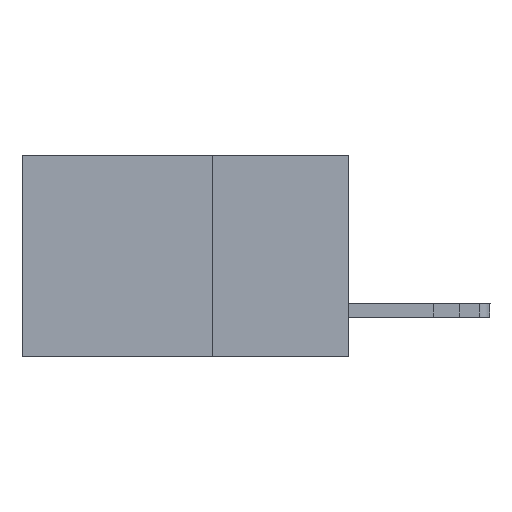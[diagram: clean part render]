
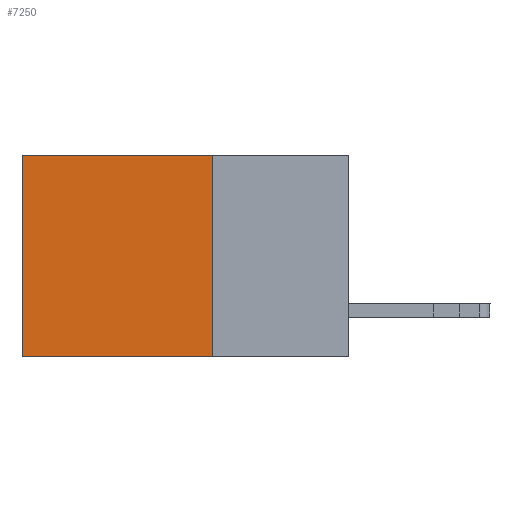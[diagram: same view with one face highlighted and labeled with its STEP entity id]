
A CAD part, left-side view. The second image highlights one B-rep face of the part: STEP entity #7250.
In plain terms, the highlighted planar face has unit normal (-1, 0, 0).
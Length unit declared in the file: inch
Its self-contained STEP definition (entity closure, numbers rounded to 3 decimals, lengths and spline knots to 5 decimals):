
#234 = DIRECTION ( 'NONE',  ( 0., 0., -1. ) ) ;
#355 = VERTEX_POINT ( 'NONE', #6419 ) ;
#730 = ORIENTED_EDGE ( 'NONE', *, *, #4278, .F. ) ;
#1530 = CARTESIAN_POINT ( 'NONE',  ( 0.2615, 0.25, -0.37 ) ) ;
#1921 = CARTESIAN_POINT ( 'NONE',  ( 0.2615, 0.25, 0. ) ) ;
#2441 = AXIS2_PLACEMENT_3D ( 'NONE', #8432, #5954, #5156 ) ;
#2687 = LINE ( 'NONE', #1921, #5431 ) ;
#2782 = PLANE ( 'NONE',  #2441 ) ;
#2874 = FACE_OUTER_BOUND ( 'NONE', #3683, .T. ) ;
#2915 = VECTOR ( 'NONE', #6944, 39.37008 ) ;
#3198 = VECTOR ( 'NONE', #234, 39.37008 ) ;
#3479 = CARTESIAN_POINT ( 'NONE',  ( 0.2615, 0.6, 0. ) ) ;
#3683 = EDGE_LOOP ( 'NONE', ( #8567, #730, #8002, #8547 ) ) ;
#3922 = CARTESIAN_POINT ( 'NONE',  ( 0.2615, 0.25, -0.37 ) ) ;
#3993 = EDGE_CURVE ( 'NONE', #6884, #7990, #2687, .T. ) ;
#4278 = EDGE_CURVE ( 'NONE', #5922, #355, #8503, .T. ) ;
#4698 = EDGE_CURVE ( 'NONE', #6884, #5922, #4733, .T. ) ;
#4733 = LINE ( 'NONE', #1530, #2915 ) ;
#4988 = LINE ( 'NONE', #8118, #3198 ) ;
#5156 = DIRECTION ( 'NONE',  ( 0., 0., -1. ) ) ;
#5431 = VECTOR ( 'NONE', #7934, 39.37008 ) ;
#5922 = VERTEX_POINT ( 'NONE', #7621 ) ;
#5954 = DIRECTION ( 'NONE',  ( 1., 0., 0. ) ) ;
#6419 = CARTESIAN_POINT ( 'NONE',  ( 0.2615, 0.6, -0.37 ) ) ;
#6884 = VERTEX_POINT ( 'NONE', #9486 ) ;
#6944 = DIRECTION ( 'NONE',  ( 0., 0., -1. ) ) ;
#7250 = ADVANCED_FACE ( 'NONE', ( #2874 ), #2782, .F. ) ;
#7621 = CARTESIAN_POINT ( 'NONE',  ( 0.2615, 0.25, -0.37 ) ) ;
#7880 = DIRECTION ( 'NONE',  ( 0., 1., 0. ) ) ;
#7934 = DIRECTION ( 'NONE',  ( 0., 1., 0. ) ) ;
#7990 = VERTEX_POINT ( 'NONE', #3479 ) ;
#8002 = ORIENTED_EDGE ( 'NONE', *, *, #4698, .F. ) ;
#8052 = VECTOR ( 'NONE', #7880, 39.37008 ) ;
#8118 = CARTESIAN_POINT ( 'NONE',  ( 0.2615, 0.6, -0.37 ) ) ;
#8432 = CARTESIAN_POINT ( 'NONE',  ( 0.2615, 0.25, -0.37 ) ) ;
#8503 = LINE ( 'NONE', #3922, #8052 ) ;
#8547 = ORIENTED_EDGE ( 'NONE', *, *, #3993, .T. ) ;
#8567 = ORIENTED_EDGE ( 'NONE', *, *, #9173, .T. ) ;
#9173 = EDGE_CURVE ( 'NONE', #7990, #355, #4988, .T. ) ;
#9486 = CARTESIAN_POINT ( 'NONE',  ( 0.2615, 0.25, 0. ) ) ;
